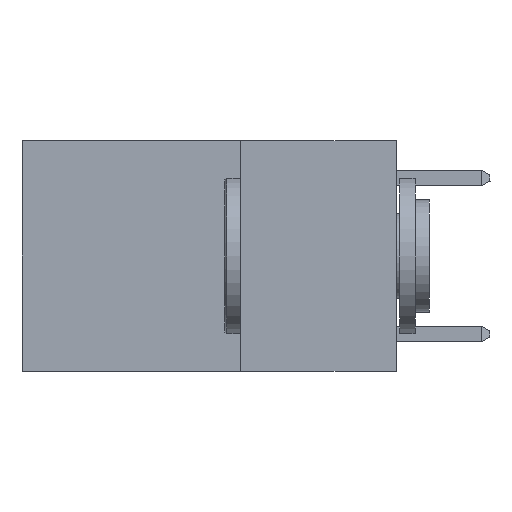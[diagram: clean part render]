
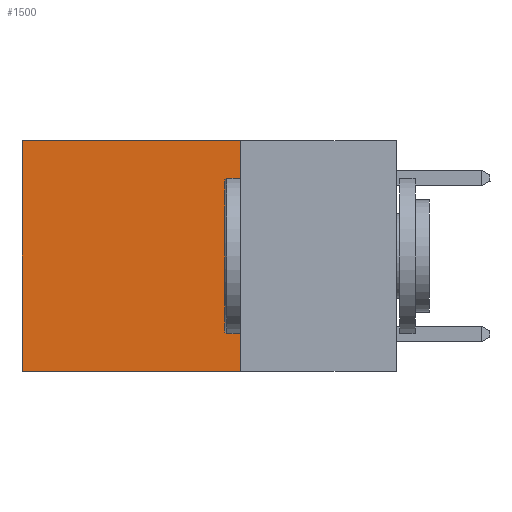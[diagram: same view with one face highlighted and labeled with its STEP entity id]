
A CAD part, left-side view. The second image highlights one B-rep face of the part: STEP entity #1500.
In plain terms, the highlighted planar face has unit normal (-1, 0, 0).
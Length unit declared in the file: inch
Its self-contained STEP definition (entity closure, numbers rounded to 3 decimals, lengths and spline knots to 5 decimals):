
#288 = DIRECTION ( 'NONE',  ( 0., 0., -1. ) ) ;
#821 = ORIENTED_EDGE ( 'NONE', *, *, #12124, .F. ) ;
#1500 = ADVANCED_FACE ( 'NONE', ( #24443 ), #10926, .F. ) ;
#1989 = LINE ( 'NONE', #27786, #9592 ) ;
#2329 = CARTESIAN_POINT ( 'NONE',  ( 0.2625, 0.25, 0. ) ) ;
#3028 = ORIENTED_EDGE ( 'NONE', *, *, #23439, .F. ) ;
#3322 = CARTESIAN_POINT ( 'NONE',  ( 0.2625, 0.6, 0. ) ) ;
#4658 = CARTESIAN_POINT ( 'NONE',  ( 0.2625, 0.25, 0. ) ) ;
#8763 = VERTEX_POINT ( 'NONE', #15126 ) ;
#8919 = VECTOR ( 'NONE', #13340, 39.37008 ) ;
#9592 = VECTOR ( 'NONE', #31349, 39.37008 ) ;
#9870 = LINE ( 'NONE', #15021, #22184 ) ;
#10634 = CARTESIAN_POINT ( 'NONE',  ( 0.2625, 0.6, -0.37 ) ) ;
#10926 = PLANE ( 'NONE',  #20627 ) ;
#11943 = ORIENTED_EDGE ( 'NONE', *, *, #13679, .T. ) ;
#12124 = EDGE_CURVE ( 'NONE', #8763, #22160, #24665, .T. ) ;
#13334 = VERTEX_POINT ( 'NONE', #3322 ) ;
#13340 = DIRECTION ( 'NONE',  ( 0., 1., 0. ) ) ;
#13679 = EDGE_CURVE ( 'NONE', #13334, #22160, #1989, .T. ) ;
#15021 = CARTESIAN_POINT ( 'NONE',  ( 0.2625, 0.25, 0. ) ) ;
#15126 = CARTESIAN_POINT ( 'NONE',  ( 0.2625, 0.25, -0.37 ) ) ;
#17739 = DIRECTION ( 'NONE',  ( 0., 1., 0. ) ) ;
#18119 = DIRECTION ( 'NONE',  ( 1., 0., 0. ) ) ;
#20029 = VECTOR ( 'NONE', #288, 39.37008 ) ;
#20596 = DIRECTION ( 'NONE',  ( 0., 0., -1. ) ) ;
#20627 = AXIS2_PLACEMENT_3D ( 'NONE', #30416, #18119, #20596 ) ;
#21538 = ORIENTED_EDGE ( 'NONE', *, *, #26227, .T. ) ;
#21648 = VERTEX_POINT ( 'NONE', #2329 ) ;
#22160 = VERTEX_POINT ( 'NONE', #10634 ) ;
#22184 = VECTOR ( 'NONE', #17739, 39.37008 ) ;
#22720 = CARTESIAN_POINT ( 'NONE',  ( 0.2625, 0.25, -0.37 ) ) ;
#23439 = EDGE_CURVE ( 'NONE', #21648, #8763, #26559, .T. ) ;
#24402 = EDGE_LOOP ( 'NONE', ( #11943, #821, #3028, #21538 ) ) ;
#24443 = FACE_OUTER_BOUND ( 'NONE', #24402, .T. ) ;
#24665 = LINE ( 'NONE', #22720, #8919 ) ;
#26227 = EDGE_CURVE ( 'NONE', #21648, #13334, #9870, .T. ) ;
#26559 = LINE ( 'NONE', #4658, #20029 ) ;
#27786 = CARTESIAN_POINT ( 'NONE',  ( 0.2625, 0.6, 0. ) ) ;
#30416 = CARTESIAN_POINT ( 'NONE',  ( 0.2625, 0.25, 0. ) ) ;
#31349 = DIRECTION ( 'NONE',  ( 0., 0., -1. ) ) ;
